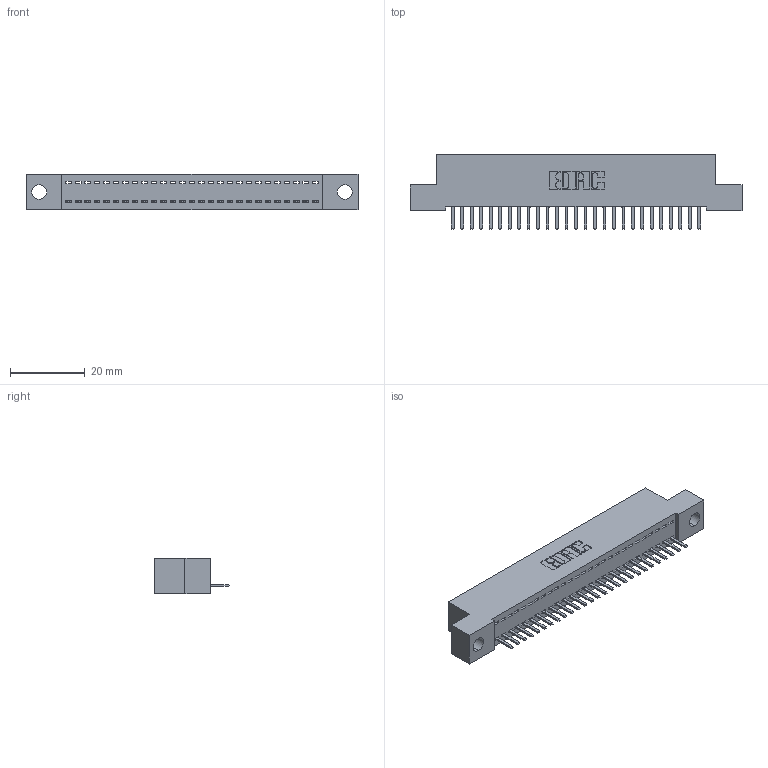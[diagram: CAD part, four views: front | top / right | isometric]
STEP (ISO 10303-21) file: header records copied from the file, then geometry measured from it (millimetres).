
FILE_DESCRIPTION (( 'STEP AP203' ), '1' );
FILE_NAME ('342-027-520-104.STEP', '2019-10-02T01:58:28', ( '' ), ( '' ), 'SwSTEP 2.0', 'SolidWorks 2016', '' );
FILE_SCHEMA (( 'CONFIG_CONTROL_DESIGN' ));
Length unit declared in the file: inch
Products named in the file (3): 345-292-001_345-293-120; 342-027-520-104; 342 Part_.156 TH
Assembly tree (28 placements, depth 2):
  342-027-520-104
    342 Part_.156 TH
    345-292-001_345-293-120  x27
Bounding box: 88.9 x 20.02 x 9.4 mm (x, y, z)
Volume: 7574.8 mm3; surface area: 10413.6 mm2
Topology: 28 solids, 28 shells, 1784 faces, 5267 edges, 3438 vertices
Faces by surface type: plane 1254, cylinder 530
Entity records: 18431 total; most frequent: CARTESIAN_POINT 3199, ORIENTED_EDGE 3150, DIRECTION 2717, EDGE_CURVE 1575, LINE 1443, VECTOR 1443, VERTEX_POINT 1046, AXIS2_PLACEMENT_3D 637
